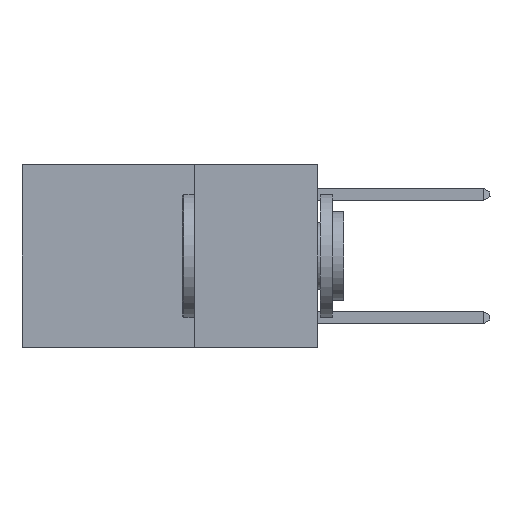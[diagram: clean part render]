
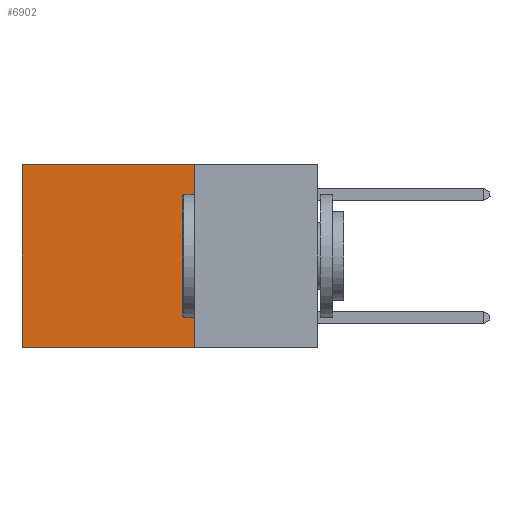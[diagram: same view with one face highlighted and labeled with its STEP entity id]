
A CAD part, left-side view. The second image highlights one B-rep face of the part: STEP entity #6902.
In plain terms, the highlighted planar face has unit normal (-1, 0, 0).
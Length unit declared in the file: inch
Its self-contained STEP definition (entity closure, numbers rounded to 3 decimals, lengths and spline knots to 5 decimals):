
#533 = AXIS2_PLACEMENT_3D ( 'NONE', #752, #3687, #9863 ) ;
#752 = CARTESIAN_POINT ( 'NONE',  ( 0.2625, 0.25, 0. ) ) ;
#753 = CARTESIAN_POINT ( 'NONE',  ( 0.2625, 0.6, 0. ) ) ;
#1636 = ORIENTED_EDGE ( 'NONE', *, *, #5982, .T. ) ;
#1778 = VERTEX_POINT ( 'NONE', #3416 ) ;
#1798 = CARTESIAN_POINT ( 'NONE',  ( 0.2625, 0.6, -0.37 ) ) ;
#2091 = ORIENTED_EDGE ( 'NONE', *, *, #3887, .F. ) ;
#2578 = LINE ( 'NONE', #5813, #7418 ) ;
#2587 = FACE_OUTER_BOUND ( 'NONE', #4503, .T. ) ;
#2801 = VECTOR ( 'NONE', #11249, 39.37008 ) ;
#3416 = CARTESIAN_POINT ( 'NONE',  ( 0.2625, 0.25, -0.37 ) ) ;
#3639 = CARTESIAN_POINT ( 'NONE',  ( 0.2625, 0.25, 0. ) ) ;
#3687 = DIRECTION ( 'NONE',  ( 1., 0., 0. ) ) ;
#3887 = EDGE_CURVE ( 'NONE', #8751, #1778, #8256, .T. ) ;
#4503 = EDGE_LOOP ( 'NONE', ( #9484, #4830, #2091, #1636 ) ) ;
#4830 = ORIENTED_EDGE ( 'NONE', *, *, #9370, .F. ) ;
#5813 = CARTESIAN_POINT ( 'NONE',  ( 0.2625, 0.6, 0. ) ) ;
#5982 = EDGE_CURVE ( 'NONE', #8751, #6035, #6161, .T. ) ;
#6035 = VERTEX_POINT ( 'NONE', #753 ) ;
#6161 = LINE ( 'NONE', #7160, #10386 ) ;
#6902 = ADVANCED_FACE ( 'NONE', ( #2587 ), #11383, .F. ) ;
#7160 = CARTESIAN_POINT ( 'NONE',  ( 0.2625, 0.25, 0. ) ) ;
#7418 = VECTOR ( 'NONE', #9200, 39.37008 ) ;
#7607 = LINE ( 'NONE', #7876, #2801 ) ;
#7786 = DIRECTION ( 'NONE',  ( 0., 0., -1. ) ) ;
#7876 = CARTESIAN_POINT ( 'NONE',  ( 0.2625, 0.25, -0.37 ) ) ;
#7934 = CARTESIAN_POINT ( 'NONE',  ( 0.2625, 0.25, 0. ) ) ;
#7977 = DIRECTION ( 'NONE',  ( 0., 1., 0. ) ) ;
#8256 = LINE ( 'NONE', #7934, #10313 ) ;
#8751 = VERTEX_POINT ( 'NONE', #3639 ) ;
#9200 = DIRECTION ( 'NONE',  ( 0., 0., -1. ) ) ;
#9370 = EDGE_CURVE ( 'NONE', #1778, #9472, #7607, .T. ) ;
#9472 = VERTEX_POINT ( 'NONE', #1798 ) ;
#9484 = ORIENTED_EDGE ( 'NONE', *, *, #10704, .T. ) ;
#9863 = DIRECTION ( 'NONE',  ( 0., 0., -1. ) ) ;
#10313 = VECTOR ( 'NONE', #7786, 39.37008 ) ;
#10386 = VECTOR ( 'NONE', #7977, 39.37008 ) ;
#10704 = EDGE_CURVE ( 'NONE', #6035, #9472, #2578, .T. ) ;
#11249 = DIRECTION ( 'NONE',  ( 0., 1., 0. ) ) ;
#11383 = PLANE ( 'NONE',  #533 ) ;
